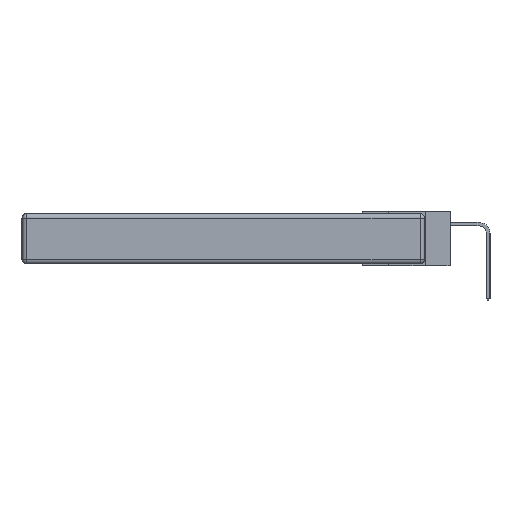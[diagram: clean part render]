
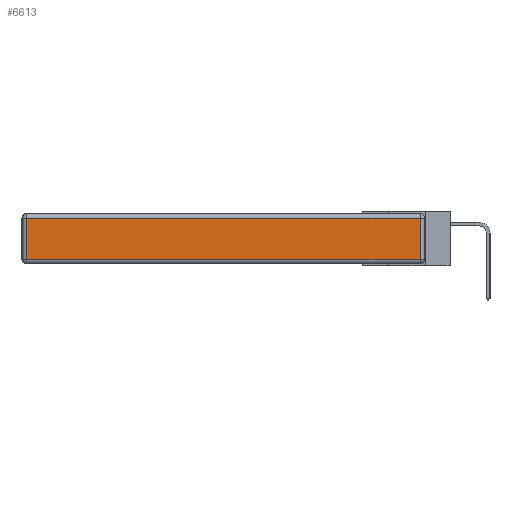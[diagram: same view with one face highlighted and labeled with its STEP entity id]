
A CAD part, left-side view. The second image highlights one B-rep face of the part: STEP entity #6613.
In plain terms, the highlighted planar face has unit normal (-1, 0, 0).
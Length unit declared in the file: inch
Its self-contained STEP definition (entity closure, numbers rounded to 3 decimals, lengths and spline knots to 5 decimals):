
#230 = CARTESIAN_POINT ( 'NONE',  ( 0., 0., -0.313 ) ) ;
#597 = LINE ( 'NONE', #11350, #8305 ) ;
#3418 = VERTEX_POINT ( 'NONE', #7295 ) ;
#4149 = CARTESIAN_POINT ( 'NONE',  ( 0., 0.03, -0.343 ) ) ;
#4161 = LINE ( 'NONE', #230, #14985 ) ;
#4562 = AXIS2_PLACEMENT_3D ( 'NONE', #5642, #10131, #14394 ) ;
#5389 = EDGE_CURVE ( 'NONE', #13813, #7231, #11961, .T. ) ;
#5642 = CARTESIAN_POINT ( 'NONE',  ( 0., 0., -0.343 ) ) ;
#6412 = VECTOR ( 'NONE', #15426, 39.37008 ) ;
#6424 = CARTESIAN_POINT ( 'NONE',  ( 0., 2.72, -0.03 ) ) ;
#6613 = ADVANCED_FACE ( 'NONE', ( #17930 ), #6760, .T. ) ;
#6760 = PLANE ( 'NONE',  #4562 ) ;
#7231 = VERTEX_POINT ( 'NONE', #6424 ) ;
#7295 = CARTESIAN_POINT ( 'NONE',  ( 0., 2.72, -0.313 ) ) ;
#8305 = VECTOR ( 'NONE', #9821, 39.37008 ) ;
#8452 = DIRECTION ( 'NONE',  ( 0., 1., 0. ) ) ;
#9821 = DIRECTION ( 'NONE',  ( 0., 0., -1. ) ) ;
#9946 = EDGE_CURVE ( 'NONE', #14406, #13813, #13683, .T. ) ;
#10131 = DIRECTION ( 'NONE',  ( -1., 0., 0. ) ) ;
#10902 = ORIENTED_EDGE ( 'NONE', *, *, #13160, .T. ) ;
#11222 = DIRECTION ( 'NONE',  ( 0., -1., 0. ) ) ;
#11275 = EDGE_CURVE ( 'NONE', #3418, #14406, #4161, .T. ) ;
#11350 = CARTESIAN_POINT ( 'NONE',  ( 0., 2.72, -0.343 ) ) ;
#11961 = LINE ( 'NONE', #14090, #12179 ) ;
#12179 = VECTOR ( 'NONE', #8452, 39.37008 ) ;
#12301 = ORIENTED_EDGE ( 'NONE', *, *, #9946, .T. ) ;
#13160 = EDGE_CURVE ( 'NONE', #7231, #3418, #597, .T. ) ;
#13683 = LINE ( 'NONE', #4149, #6412 ) ;
#13813 = VERTEX_POINT ( 'NONE', #14311 ) ;
#14090 = CARTESIAN_POINT ( 'NONE',  ( 0., 2.75, -0.03 ) ) ;
#14311 = CARTESIAN_POINT ( 'NONE',  ( 0., 0.03, -0.03 ) ) ;
#14394 = DIRECTION ( 'NONE',  ( 0., 0., 1. ) ) ;
#14406 = VERTEX_POINT ( 'NONE', #16953 ) ;
#14985 = VECTOR ( 'NONE', #11222, 39.37008 ) ;
#15426 = DIRECTION ( 'NONE',  ( 0., 0., 1. ) ) ;
#15527 = ORIENTED_EDGE ( 'NONE', *, *, #5389, .T. ) ;
#16953 = CARTESIAN_POINT ( 'NONE',  ( 0., 0.03, -0.313 ) ) ;
#17184 = EDGE_LOOP ( 'NONE', ( #18048, #12301, #15527, #10902 ) ) ;
#17930 = FACE_OUTER_BOUND ( 'NONE', #17184, .T. ) ;
#18048 = ORIENTED_EDGE ( 'NONE', *, *, #11275, .T. ) ;
